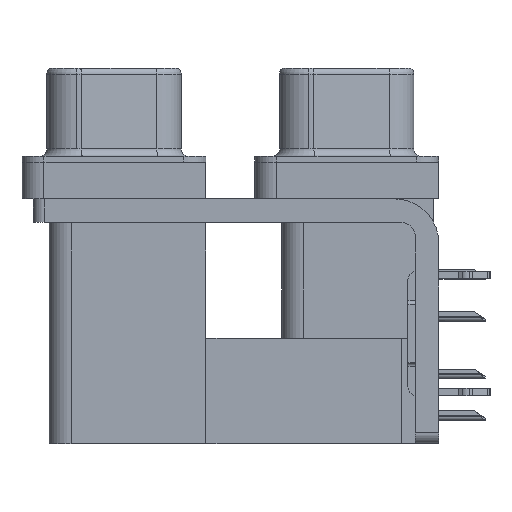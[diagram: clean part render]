
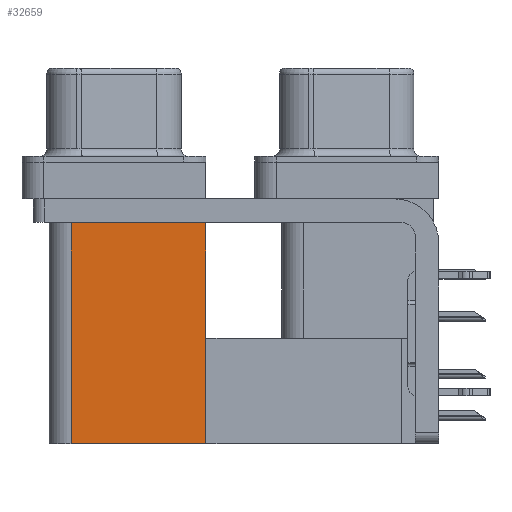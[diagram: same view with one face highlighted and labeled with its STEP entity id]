
A CAD part, left-side view. The second image highlights one B-rep face of the part: STEP entity #32659.
In plain terms, the highlighted planar face has unit normal (-1, 0, 0).
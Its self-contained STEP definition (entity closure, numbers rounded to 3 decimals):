
#380 = LINE ( 'NONE', #27091, #35642 ) ;
#2895 = ORIENTED_EDGE ( 'NONE', *, *, #3316, .T. ) ;
#3316 = EDGE_CURVE ( 'NONE', #38378, #11625, #36438, .T. ) ;
#6318 = VERTEX_POINT ( 'NONE', #16620 ) ;
#7157 = DIRECTION ( 'NONE',  ( 1., 0., 0. ) ) ;
#8695 = CARTESIAN_POINT ( 'NONE',  ( 3.7, 9.6, -2.5 ) ) ;
#9554 = PLANE ( 'NONE',  #37131 ) ;
#9564 = VECTOR ( 'NONE', #39697, 1000. ) ;
#11039 = CARTESIAN_POINT ( 'NONE',  ( 3.7, 18.8, -19.2 ) ) ;
#11260 = EDGE_CURVE ( 'NONE', #17480, #6318, #25442, .T. ) ;
#11625 = VERTEX_POINT ( 'NONE', #30496 ) ;
#12790 = DIRECTION ( 'NONE',  ( 0., 1., 0. ) ) ;
#14820 = DIRECTION ( 'NONE',  ( 0., 0., 1. ) ) ;
#16074 = VECTOR ( 'NONE', #12790, 1000. ) ;
#16278 = FACE_OUTER_BOUND ( 'NONE', #39273, .T. ) ;
#16620 = CARTESIAN_POINT ( 'NONE',  ( 3.7, 18.8, -2.5 ) ) ;
#17090 = CARTESIAN_POINT ( 'NONE',  ( 3.7, 9.6, -19.2 ) ) ;
#17480 = VERTEX_POINT ( 'NONE', #11039 ) ;
#18914 = CARTESIAN_POINT ( 'NONE',  ( 3.7, 18.8, -19.2 ) ) ;
#19399 = ORIENTED_EDGE ( 'NONE', *, *, #27114, .T. ) ;
#22416 = ORIENTED_EDGE ( 'NONE', *, *, #11260, .F. ) ;
#23440 = CARTESIAN_POINT ( 'NONE',  ( 3.7, 9.6, -19.2 ) ) ;
#24848 = CARTESIAN_POINT ( 'NONE',  ( 3.7, 9.6, -19.2 ) ) ;
#25442 = LINE ( 'NONE', #18914, #37195 ) ;
#27091 = CARTESIAN_POINT ( 'NONE',  ( 3.7, 9.6, -19.2 ) ) ;
#27114 = EDGE_CURVE ( 'NONE', #11625, #6318, #35001, .T. ) ;
#27522 = DIRECTION ( 'NONE',  ( 0., 1., 0. ) ) ;
#28787 = ORIENTED_EDGE ( 'NONE', *, *, #31407, .F. ) ;
#30496 = CARTESIAN_POINT ( 'NONE',  ( 3.7, 9.6, -2.5 ) ) ;
#31407 = EDGE_CURVE ( 'NONE', #38378, #17480, #380, .T. ) ;
#32659 = ADVANCED_FACE ( 'NONE', ( #16278 ), #9554, .F. ) ;
#35001 = LINE ( 'NONE', #8695, #16074 ) ;
#35642 = VECTOR ( 'NONE', #27522, 1000. ) ;
#36438 = LINE ( 'NONE', #17090, #9564 ) ;
#36692 = DIRECTION ( 'NONE',  ( 0., 0., -1. ) ) ;
#37131 = AXIS2_PLACEMENT_3D ( 'NONE', #23440, #7157, #36692 ) ;
#37195 = VECTOR ( 'NONE', #14820, 1000. ) ;
#38378 = VERTEX_POINT ( 'NONE', #24848 ) ;
#39273 = EDGE_LOOP ( 'NONE', ( #19399, #22416, #28787, #2895 ) ) ;
#39697 = DIRECTION ( 'NONE',  ( 0., 0., 1. ) ) ;
